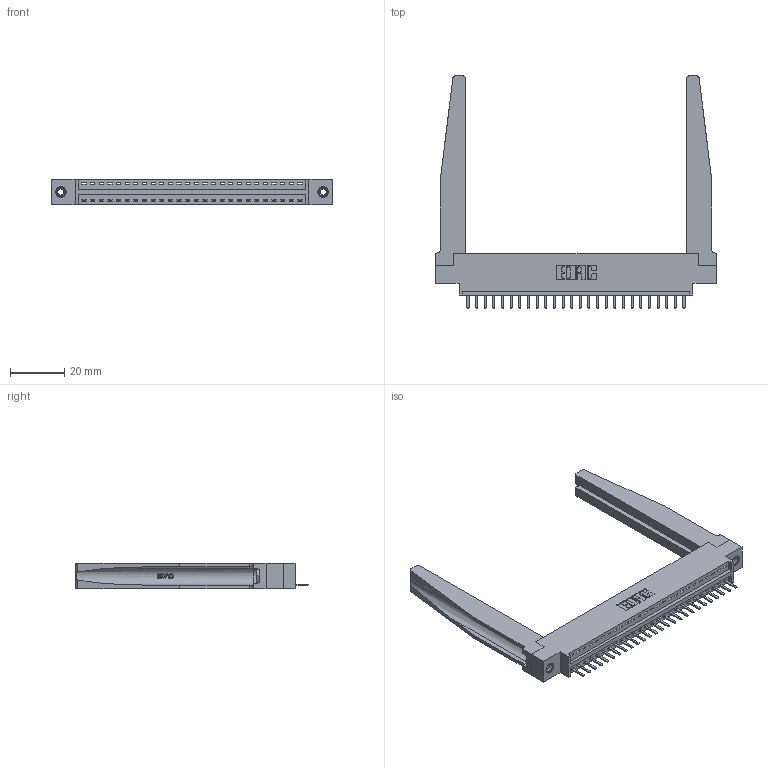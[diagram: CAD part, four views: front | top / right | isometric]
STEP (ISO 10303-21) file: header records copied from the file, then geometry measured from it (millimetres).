
FILE_DESCRIPTION (( 'STEP AP203' ), '1' );
FILE_NAME ('396-026-520-678.STEP', '2019-10-27T06:58:54', ( '' ), ( '' ), 'SwSTEP 2.0', 'SolidWorks 2016', '' );
FILE_SCHEMA (( 'CONFIG_CONTROL_DESIGN' ));
Length unit declared in the file: inch
Products named in the file (5): 346-220-078_345-220-078; 345-292-001_345-293-120; 345-250-001_345-250-001-102; 396-026-520-678; 346 Part_0.170 Offset - 0.156 Dia-TH
Assembly tree (31 placements, depth 2):
  396-026-520-678
    346 Part_0.170 Offset - 0.156 Dia-TH
    345-292-001_345-293-120  x26
    346-220-078_345-220-078  x2
    345-250-001_345-250-001-102  x2
Bounding box: 103.12 x 85.29 x 9.4 mm (x, y, z)
Volume: 16440.5 mm3; surface area: 18191.4 mm2
Topology: 31 solids, 31 shells, 1972 faces, 5733 edges, 3742 vertices
Faces by surface type: plane 1314, cylinder 606, bspline 36, cone 12, torus 4
Entity records: 23284 total; most frequent: CARTESIAN_POINT 4921, ORIENTED_EDGE 3758, DIRECTION 3333, EDGE_CURVE 1879, LINE 1545, VECTOR 1545, VERTEX_POINT 1244, AXIS2_PLACEMENT_3D 894
